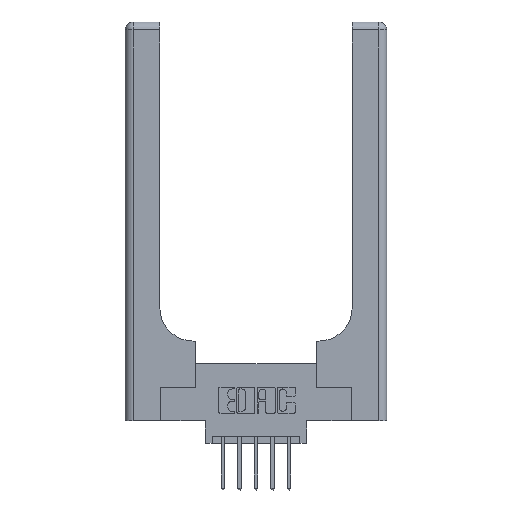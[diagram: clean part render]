
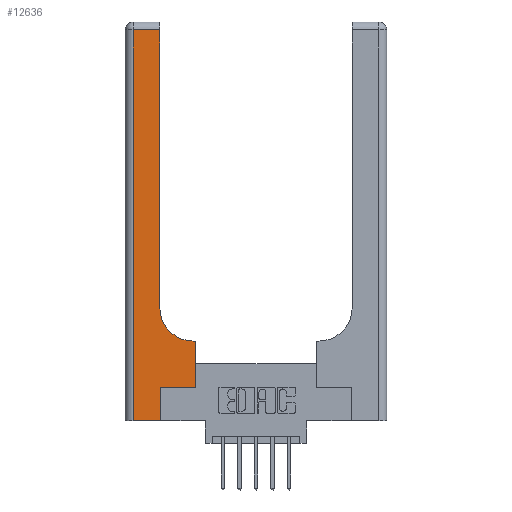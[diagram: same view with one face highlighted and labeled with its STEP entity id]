
A CAD part, top view. The second image highlights one B-rep face of the part: STEP entity #12636.
In plain terms, the highlighted planar face has unit normal (0, 0, 1).
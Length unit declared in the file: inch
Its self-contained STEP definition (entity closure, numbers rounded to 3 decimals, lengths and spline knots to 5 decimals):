
#19 = PLANE ( 'NONE',  #2578 ) ;
#42 = EDGE_CURVE ( 'NONE', #7049, #721, #9749, .T. ) ;
#53 = DIRECTION ( 'NONE',  ( 1., 0., 0. ) ) ;
#515 = VECTOR ( 'NONE', #3907, 39.37008 ) ;
#721 = VERTEX_POINT ( 'NONE', #8701 ) ;
#738 = CARTESIAN_POINT ( 'NONE',  ( 0.06, 0., 0.37 ) ) ;
#781 = DIRECTION ( 'NONE',  ( -1., 0., 0. ) ) ;
#852 = LINE ( 'NONE', #6336, #1167 ) ;
#938 = EDGE_CURVE ( 'NONE', #5574, #8058, #6969, .T. ) ;
#968 = CARTESIAN_POINT ( 'NONE',  ( 0.265, 0., 0.37 ) ) ;
#969 = VERTEX_POINT ( 'NONE', #7004 ) ;
#1066 = CARTESIAN_POINT ( 'NONE',  ( 0., 3., 0.37 ) ) ;
#1167 = VECTOR ( 'NONE', #53, 39.37008 ) ;
#1180 = EDGE_CURVE ( 'NONE', #6297, #5574, #7455, .T. ) ;
#1185 = CARTESIAN_POINT ( 'NONE',  ( 0.26, 0.85, 0.37 ) ) ;
#1227 = ORIENTED_EDGE ( 'NONE', *, *, #42, .T. ) ;
#1545 = FACE_OUTER_BOUND ( 'NONE', #11019, .T. ) ;
#1606 = CARTESIAN_POINT ( 'NONE',  ( 0.26, 2.94, 0.37 ) ) ;
#1635 = VECTOR ( 'NONE', #10453, 39.37008 ) ;
#1819 = ORIENTED_EDGE ( 'NONE', *, *, #5754, .T. ) ;
#2110 = DIRECTION ( 'NONE',  ( 0., 0., -1. ) ) ;
#2162 = LINE ( 'NONE', #5999, #7427 ) ;
#2185 = EDGE_CURVE ( 'NONE', #9151, #7049, #9753, .T. ) ;
#2578 = AXIS2_PLACEMENT_3D ( 'NONE', #1066, #2110, #9474 ) ;
#2851 = CARTESIAN_POINT ( 'NONE',  ( 0.06, 3., 0.37 ) ) ;
#2909 = CARTESIAN_POINT ( 'NONE',  ( 0.26, 3., 0.37 ) ) ;
#3069 = CARTESIAN_POINT ( 'NONE',  ( 0.265, 0., 0.37 ) ) ;
#3358 = CIRCLE ( 'NONE', #12119, 0.25 ) ;
#3453 = CARTESIAN_POINT ( 'NONE',  ( 0.528, 0.6, 0.37 ) ) ;
#3464 = CARTESIAN_POINT ( 'NONE',  ( 0.51, 0.6, 0.37 ) ) ;
#3498 = EDGE_CURVE ( 'NONE', #969, #6297, #852, .T. ) ;
#3564 = ORIENTED_EDGE ( 'NONE', *, *, #10255, .T. ) ;
#3611 = LINE ( 'NONE', #2851, #515 ) ;
#3762 = ORIENTED_EDGE ( 'NONE', *, *, #1180, .T. ) ;
#3907 = DIRECTION ( 'NONE',  ( 0., -1., 0. ) ) ;
#4148 = VECTOR ( 'NONE', #9074, 39.37008 ) ;
#4756 = CARTESIAN_POINT ( 'NONE',  ( 0.51, 0.85, 0.37 ) ) ;
#4877 = ORIENTED_EDGE ( 'NONE', *, *, #3498, .T. ) ;
#4970 = DIRECTION ( 'NONE',  ( 1., 0., 0. ) ) ;
#5021 = ORIENTED_EDGE ( 'NONE', *, *, #938, .T. ) ;
#5336 = ORIENTED_EDGE ( 'NONE', *, *, #10097, .T. ) ;
#5404 = ORIENTED_EDGE ( 'NONE', *, *, #2185, .T. ) ;
#5574 = VERTEX_POINT ( 'NONE', #3453 ) ;
#5754 = EDGE_CURVE ( 'NONE', #8058, #9151, #3358, .T. ) ;
#5827 = DIRECTION ( 'NONE',  ( 1., 0., 0. ) ) ;
#5998 = CARTESIAN_POINT ( 'NONE',  ( 0., 2.94, 0.37 ) ) ;
#5999 = CARTESIAN_POINT ( 'NONE',  ( 0., 0., 0.37 ) ) ;
#6297 = VERTEX_POINT ( 'NONE', #12930 ) ;
#6336 = CARTESIAN_POINT ( 'NONE',  ( 0.265, 0.25, 0.37 ) ) ;
#6969 = LINE ( 'NONE', #12214, #4148 ) ;
#7004 = CARTESIAN_POINT ( 'NONE',  ( 0.265, 0.25, 0.37 ) ) ;
#7049 = VERTEX_POINT ( 'NONE', #1606 ) ;
#7427 = VECTOR ( 'NONE', #4970, 39.37008 ) ;
#7455 = LINE ( 'NONE', #9484, #12411 ) ;
#7618 = VERTEX_POINT ( 'NONE', #738 ) ;
#7640 = EDGE_CURVE ( 'NONE', #7618, #13247, #2162, .T. ) ;
#8058 = VERTEX_POINT ( 'NONE', #3464 ) ;
#8701 = CARTESIAN_POINT ( 'NONE',  ( 0.06, 2.94, 0.37 ) ) ;
#9074 = DIRECTION ( 'NONE',  ( -1., 0., 0. ) ) ;
#9151 = VERTEX_POINT ( 'NONE', #1185 ) ;
#9474 = DIRECTION ( 'NONE',  ( -1., 0., 0. ) ) ;
#9484 = CARTESIAN_POINT ( 'NONE',  ( 0.528, 0.25, 0.37 ) ) ;
#9694 = LINE ( 'NONE', #3069, #1635 ) ;
#9749 = LINE ( 'NONE', #5998, #11902 ) ;
#9753 = LINE ( 'NONE', #2909, #10098 ) ;
#10097 = EDGE_CURVE ( 'NONE', #721, #7618, #3611, .T. ) ;
#10098 = VECTOR ( 'NONE', #10304, 39.37008 ) ;
#10255 = EDGE_CURVE ( 'NONE', #13247, #969, #9694, .T. ) ;
#10304 = DIRECTION ( 'NONE',  ( 0., 1., 0. ) ) ;
#10382 = DIRECTION ( 'NONE',  ( 0., 1., 0. ) ) ;
#10453 = DIRECTION ( 'NONE',  ( 0., 1., 0. ) ) ;
#10521 = ORIENTED_EDGE ( 'NONE', *, *, #7640, .T. ) ;
#11019 = EDGE_LOOP ( 'NONE', ( #5404, #1227, #5336, #10521, #3564, #4877, #3762, #5021, #1819 ) ) ;
#11902 = VECTOR ( 'NONE', #781, 39.37008 ) ;
#12119 = AXIS2_PLACEMENT_3D ( 'NONE', #4756, #12168, #5827 ) ;
#12168 = DIRECTION ( 'NONE',  ( 0., 0., -1. ) ) ;
#12214 = CARTESIAN_POINT ( 'NONE',  ( 0.26, 0.6, 0.37 ) ) ;
#12411 = VECTOR ( 'NONE', #10382, 39.37008 ) ;
#12636 = ADVANCED_FACE ( 'NONE', ( #1545 ), #19, .F. ) ;
#12930 = CARTESIAN_POINT ( 'NONE',  ( 0.528, 0.25, 0.37 ) ) ;
#13247 = VERTEX_POINT ( 'NONE', #968 ) ;
